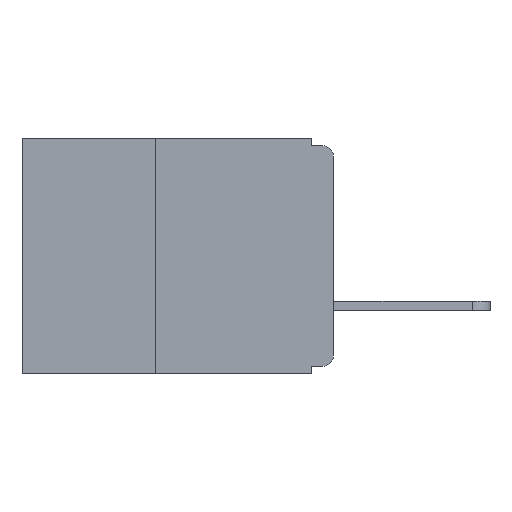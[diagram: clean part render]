
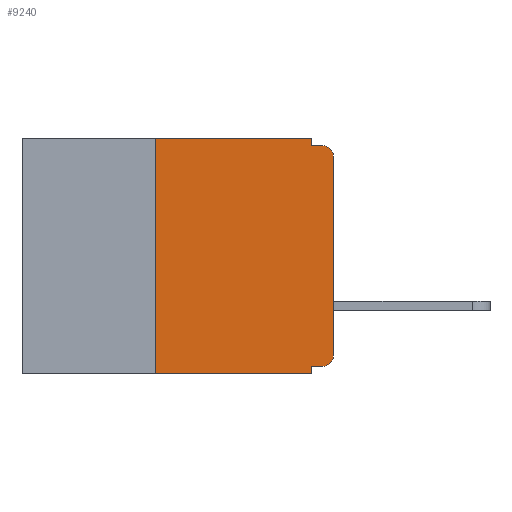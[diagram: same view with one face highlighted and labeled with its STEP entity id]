
A CAD part, left-side view. The second image highlights one B-rep face of the part: STEP entity #9240.
In plain terms, the highlighted planar face has unit normal (-1, 0, 0).
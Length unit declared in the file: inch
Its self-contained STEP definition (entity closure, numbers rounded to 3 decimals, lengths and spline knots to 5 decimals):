
#2 = ORIENTED_EDGE ( 'NONE', *, *, #11328, .F. ) ;
#200 = ORIENTED_EDGE ( 'NONE', *, *, #8446, .F. ) ;
#212 = CARTESIAN_POINT ( 'NONE',  ( 0., 0.015, -0.305 ) ) ;
#415 = EDGE_CURVE ( 'NONE', #8192, #2518, #5201, .T. ) ;
#562 = VERTEX_POINT ( 'NONE', #7340 ) ;
#564 = VERTEX_POINT ( 'NONE', #9178 ) ;
#619 = VERTEX_POINT ( 'NONE', #5531 ) ;
#633 = DIRECTION ( 'NONE',  ( 0., -1., 0. ) ) ;
#643 = CARTESIAN_POINT ( 'NONE',  ( 0., 0., 0. ) ) ;
#777 = ORIENTED_EDGE ( 'NONE', *, *, #1569, .F. ) ;
#986 = CARTESIAN_POINT ( 'NONE',  ( 0., 0.015, -0.01 ) ) ;
#1117 = DIRECTION ( 'NONE',  ( -1., 0., 0. ) ) ;
#1332 = EDGE_CURVE ( 'NONE', #562, #3833, #9887, .T. ) ;
#1569 = EDGE_CURVE ( 'NONE', #11567, #11717, #7037, .T. ) ;
#1590 = DIRECTION ( 'NONE',  ( 0., 0., -1. ) ) ;
#2001 = CARTESIAN_POINT ( 'NONE',  ( 0., 0., -0.01 ) ) ;
#2115 = CARTESIAN_POINT ( 'NONE',  ( 0., 0.015, -0.025 ) ) ;
#2173 = LINE ( 'NONE', #2268, #3592 ) ;
#2228 = DIRECTION ( 'NONE',  ( 0., 1., 0. ) ) ;
#2268 = CARTESIAN_POINT ( 'NONE',  ( 0., 0., -0.32 ) ) ;
#2393 = CARTESIAN_POINT ( 'NONE',  ( 0., 0.031, -0.01 ) ) ;
#2518 = VERTEX_POINT ( 'NONE', #6085 ) ;
#3023 = AXIS2_PLACEMENT_3D ( 'NONE', #212, #1117, #11227 ) ;
#3061 = CARTESIAN_POINT ( 'NONE',  ( 0., 0.031, 0. ) ) ;
#3414 = CARTESIAN_POINT ( 'NONE',  ( 0., 0., -0.305 ) ) ;
#3432 = CARTESIAN_POINT ( 'NONE',  ( 0., 0.031, -0.33 ) ) ;
#3592 = VECTOR ( 'NONE', #2228, 39.37008 ) ;
#3698 = VECTOR ( 'NONE', #8686, 39.37008 ) ;
#3730 = CARTESIAN_POINT ( 'NONE',  ( 0., 0.25, 0. ) ) ;
#3833 = VERTEX_POINT ( 'NONE', #10971 ) ;
#3877 = CARTESIAN_POINT ( 'NONE',  ( 0., 0., -0.025 ) ) ;
#4138 = DIRECTION ( 'NONE',  ( 0., 0., 1. ) ) ;
#4169 = CARTESIAN_POINT ( 'NONE',  ( 0., 0.437, -0.33 ) ) ;
#4296 = PLANE ( 'NONE',  #7726 ) ;
#4629 = EDGE_LOOP ( 'NONE', ( #10841, #7826, #777, #2, #7926, #5816, #5050, #5688, #200, #6454 ) ) ;
#4633 = FACE_OUTER_BOUND ( 'NONE', #4629, .T. ) ;
#4734 = CIRCLE ( 'NONE', #5120, 0.015 ) ;
#4762 = DIRECTION ( 'NONE',  ( 0., -1., 0. ) ) ;
#4966 = VECTOR ( 'NONE', #9091, 39.37008 ) ;
#5050 = ORIENTED_EDGE ( 'NONE', *, *, #7389, .T. ) ;
#5120 = AXIS2_PLACEMENT_3D ( 'NONE', #2115, #7529, #7651 ) ;
#5201 = LINE ( 'NONE', #5348, #6920 ) ;
#5261 = EDGE_CURVE ( 'NONE', #619, #8192, #10872, .T. ) ;
#5348 = CARTESIAN_POINT ( 'NONE',  ( 0., 0.437, 0. ) ) ;
#5531 = CARTESIAN_POINT ( 'NONE',  ( 0., 0.25, -0.33 ) ) ;
#5642 = LINE ( 'NONE', #4169, #5929 ) ;
#5688 = ORIENTED_EDGE ( 'NONE', *, *, #1332, .F. ) ;
#5762 = CIRCLE ( 'NONE', #3023, 0.015 ) ;
#5816 = ORIENTED_EDGE ( 'NONE', *, *, #5261, .F. ) ;
#5929 = VECTOR ( 'NONE', #633, 39.37008 ) ;
#5958 = VERTEX_POINT ( 'NONE', #3877 ) ;
#6085 = CARTESIAN_POINT ( 'NONE',  ( 0., 0.031, 0. ) ) ;
#6176 = LINE ( 'NONE', #3061, #3698 ) ;
#6454 = ORIENTED_EDGE ( 'NONE', *, *, #8392, .T. ) ;
#6920 = VECTOR ( 'NONE', #10852, 39.37008 ) ;
#7037 = LINE ( 'NONE', #2001, #11631 ) ;
#7073 = CARTESIAN_POINT ( 'NONE',  ( 0., 0.437, 0. ) ) ;
#7179 = LINE ( 'NONE', #643, #11483 ) ;
#7250 = CARTESIAN_POINT ( 'NONE',  ( 0., 0.25, -0.33 ) ) ;
#7340 = CARTESIAN_POINT ( 'NONE',  ( 0., 0.031, -0.32 ) ) ;
#7389 = EDGE_CURVE ( 'NONE', #619, #3833, #5642, .T. ) ;
#7529 = DIRECTION ( 'NONE',  ( -1., 0., 0. ) ) ;
#7651 = DIRECTION ( 'NONE',  ( 0., 0., -1. ) ) ;
#7726 = AXIS2_PLACEMENT_3D ( 'NONE', #7073, #8991, #1590 ) ;
#7826 = ORIENTED_EDGE ( 'NONE', *, *, #10694, .T. ) ;
#7926 = ORIENTED_EDGE ( 'NONE', *, *, #415, .F. ) ;
#8192 = VERTEX_POINT ( 'NONE', #3730 ) ;
#8392 = EDGE_CURVE ( 'NONE', #564, #11696, #5762, .T. ) ;
#8446 = EDGE_CURVE ( 'NONE', #564, #562, #2173, .T. ) ;
#8686 = DIRECTION ( 'NONE',  ( 0., 0., -1. ) ) ;
#8991 = DIRECTION ( 'NONE',  ( 1., 0., 0. ) ) ;
#9091 = DIRECTION ( 'NONE',  ( 0., 0., 1. ) ) ;
#9178 = CARTESIAN_POINT ( 'NONE',  ( 0., 0.015, -0.32 ) ) ;
#9240 = ADVANCED_FACE ( 'NONE', ( #4633 ), #4296, .F. ) ;
#9887 = LINE ( 'NONE', #3432, #10773 ) ;
#10694 = EDGE_CURVE ( 'NONE', #5958, #11717, #4734, .T. ) ;
#10773 = VECTOR ( 'NONE', #11710, 39.37008 ) ;
#10841 = ORIENTED_EDGE ( 'NONE', *, *, #11509, .T. ) ;
#10852 = DIRECTION ( 'NONE',  ( 0., -1., 0. ) ) ;
#10872 = LINE ( 'NONE', #7250, #4966 ) ;
#10971 = CARTESIAN_POINT ( 'NONE',  ( 0., 0.031, -0.33 ) ) ;
#11227 = DIRECTION ( 'NONE',  ( 0., 0., -1. ) ) ;
#11328 = EDGE_CURVE ( 'NONE', #2518, #11567, #6176, .T. ) ;
#11483 = VECTOR ( 'NONE', #4138, 39.37008 ) ;
#11509 = EDGE_CURVE ( 'NONE', #11696, #5958, #7179, .T. ) ;
#11567 = VERTEX_POINT ( 'NONE', #2393 ) ;
#11631 = VECTOR ( 'NONE', #4762, 39.37008 ) ;
#11696 = VERTEX_POINT ( 'NONE', #3414 ) ;
#11710 = DIRECTION ( 'NONE',  ( 0., 0., -1. ) ) ;
#11717 = VERTEX_POINT ( 'NONE', #986 ) ;
